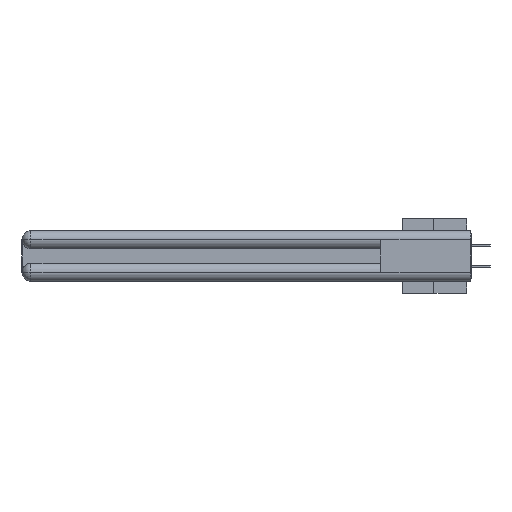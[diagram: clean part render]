
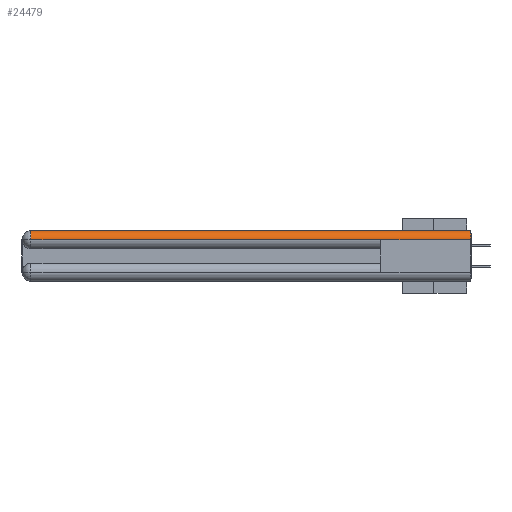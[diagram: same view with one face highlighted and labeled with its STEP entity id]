
A CAD part, left-side view. The second image highlights one B-rep face of the part: STEP entity #24479.
In plain terms, the highlighted cylindrical face has radius 1.562 mm (diameter 3.124 mm), a partial arc.
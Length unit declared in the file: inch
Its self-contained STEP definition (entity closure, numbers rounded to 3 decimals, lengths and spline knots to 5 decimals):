
#1071 = VERTEX_POINT ( 'NONE', #28728 ) ;
#1524 = CARTESIAN_POINT ( 'NONE',  ( 0.0615, 2.94, -0.0615 ) ) ;
#3821 = CARTESIAN_POINT ( 'NONE',  ( 0., 0.6, -0.0615 ) ) ;
#3867 = DIRECTION ( 'NONE',  ( 0., 0., 1. ) ) ;
#6129 = AXIS2_PLACEMENT_3D ( 'NONE', #23783, #17638, #3867 ) ;
#7412 = CARTESIAN_POINT ( 'NONE',  ( 0.0615, 0., -0.0615 ) ) ;
#8360 = DIRECTION ( 'NONE',  ( 0., 0., 1. ) ) ;
#8377 = AXIS2_PLACEMENT_3D ( 'NONE', #1524, #11573, #8360 ) ;
#8973 = EDGE_CURVE ( 'NONE', #37785, #42759, #43033, .T. ) ;
#10854 = CIRCLE ( 'NONE', #39972, 0.0615 ) ;
#11573 = DIRECTION ( 'NONE',  ( 0., -1., 0. ) ) ;
#13772 = ORIENTED_EDGE ( 'NONE', *, *, #18625, .F. ) ;
#16433 = CIRCLE ( 'NONE', #8377, 0.0615 ) ;
#16657 = ORIENTED_EDGE ( 'NONE', *, *, #26814, .F. ) ;
#17638 = DIRECTION ( 'NONE',  ( 0., 1., 0. ) ) ;
#18021 = VECTOR ( 'NONE', #24109, 39.37008 ) ;
#18625 = EDGE_CURVE ( 'NONE', #1071, #42759, #24834, .T. ) ;
#18645 = DIRECTION ( 'NONE',  ( 0., -1., 0. ) ) ;
#19538 = DIRECTION ( 'NONE',  ( 0., -1., 0. ) ) ;
#20392 = DIRECTION ( 'NONE',  ( 0., -1., 0. ) ) ;
#20937 = FACE_OUTER_BOUND ( 'NONE', #30717, .T. ) ;
#23032 = EDGE_CURVE ( 'NONE', #30510, #39824, #42478, .T. ) ;
#23783 = CARTESIAN_POINT ( 'NONE',  ( 0.0615, 0., -0.0615 ) ) ;
#24109 = DIRECTION ( 'NONE',  ( 0., 1., 0. ) ) ;
#24479 = ADVANCED_FACE ( 'NONE', ( #20937 ), #31346, .T. ) ;
#24834 = LINE ( 'NONE', #33919, #18021 ) ;
#26814 = EDGE_CURVE ( 'NONE', #39824, #1071, #10854, .T. ) ;
#27078 = CARTESIAN_POINT ( 'NONE',  ( 0.0615, 2.94, 0. ) ) ;
#28728 = CARTESIAN_POINT ( 'NONE',  ( 0., 0., -0.0615 ) ) ;
#29356 = CARTESIAN_POINT ( 'NONE',  ( 0.0615, 0., 0. ) ) ;
#29363 = ORIENTED_EDGE ( 'NONE', *, *, #8973, .T. ) ;
#30491 = DIRECTION ( 'NONE',  ( 1., 0., 0. ) ) ;
#30510 = VERTEX_POINT ( 'NONE', #27078 ) ;
#30717 = EDGE_LOOP ( 'NONE', ( #39161, #37324, #29363, #13772, #16657 ) ) ;
#31028 = CARTESIAN_POINT ( 'NONE',  ( 0., 2.94, -0.0615 ) ) ;
#31346 = CYLINDRICAL_SURFACE ( 'NONE', #6129, 0.0615 ) ;
#33457 = EDGE_CURVE ( 'NONE', #30510, #37785, #16433, .T. ) ;
#33919 = CARTESIAN_POINT ( 'NONE',  ( 0., 3., -0.0615 ) ) ;
#34192 = VECTOR ( 'NONE', #18645, 39.37008 ) ;
#36217 = VECTOR ( 'NONE', #19538, 39.37008 ) ;
#37324 = ORIENTED_EDGE ( 'NONE', *, *, #33457, .T. ) ;
#37785 = VERTEX_POINT ( 'NONE', #31028 ) ;
#38922 = CARTESIAN_POINT ( 'NONE',  ( 0., 3., -0.0615 ) ) ;
#39161 = ORIENTED_EDGE ( 'NONE', *, *, #23032, .F. ) ;
#39824 = VERTEX_POINT ( 'NONE', #42101 ) ;
#39972 = AXIS2_PLACEMENT_3D ( 'NONE', #7412, #20392, #30491 ) ;
#42101 = CARTESIAN_POINT ( 'NONE',  ( 0.0615, 0., 0. ) ) ;
#42478 = LINE ( 'NONE', #29356, #36217 ) ;
#42759 = VERTEX_POINT ( 'NONE', #3821 ) ;
#43033 = LINE ( 'NONE', #38922, #34192 ) ;
